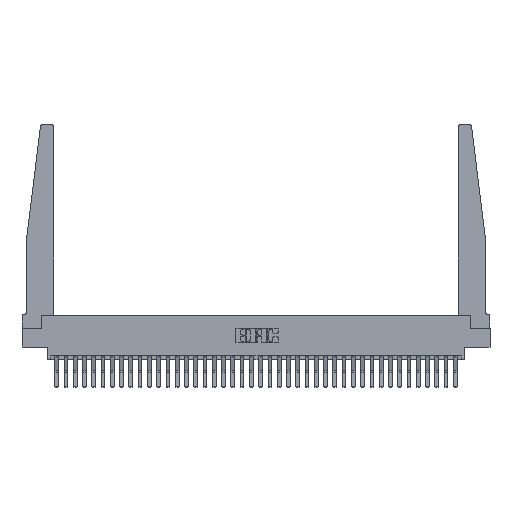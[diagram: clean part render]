
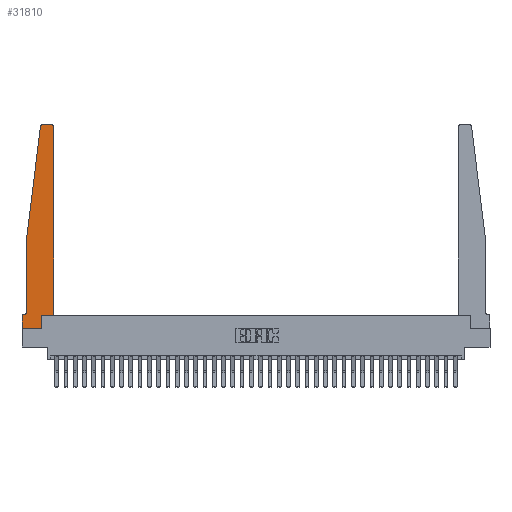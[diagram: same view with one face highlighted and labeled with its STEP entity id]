
A CAD part, top view. The second image highlights one B-rep face of the part: STEP entity #31810.
In plain terms, the highlighted planar face has unit normal (0, 0, 1).
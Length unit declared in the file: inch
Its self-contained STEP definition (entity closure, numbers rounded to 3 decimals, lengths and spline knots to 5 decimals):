
#384 = CARTESIAN_POINT ( 'NONE',  ( 0.2605, 0.18, 0.37 ) ) ;
#473 = DIRECTION ( 'NONE',  ( 1., 0., 0. ) ) ;
#571 = DIRECTION ( 'NONE',  ( 0., 0., -1. ) ) ;
#691 = AXIS2_PLACEMENT_3D ( 'NONE', #31772, #22110, #6333 ) ;
#906 = EDGE_CURVE ( 'NONE', #6547, #15479, #16368, .T. ) ;
#1162 = VERTEX_POINT ( 'NONE', #28659 ) ;
#2489 = LINE ( 'NONE', #23412, #5762 ) ;
#2725 = CARTESIAN_POINT ( 'NONE',  ( 0.27653, 2.75, 0.37 ) ) ;
#2829 = CARTESIAN_POINT ( 'NONE',  ( 0., 0., 0.37 ) ) ;
#3118 = EDGE_CURVE ( 'NONE', #28521, #12456, #17120, .T. ) ;
#3386 = VERTEX_POINT ( 'NONE', #4749 ) ;
#3524 = DIRECTION ( 'NONE',  ( 0., -1., 0. ) ) ;
#3864 = LINE ( 'NONE', #14000, #23705 ) ;
#3936 = EDGE_CURVE ( 'NONE', #12456, #9022, #10073, .T. ) ;
#4135 = VERTEX_POINT ( 'NONE', #10928 ) ;
#4567 = EDGE_CURVE ( 'NONE', #3386, #16780, #18551, .T. ) ;
#4601 = AXIS2_PLACEMENT_3D ( 'NONE', #26708, #16242, #473 ) ;
#4749 = CARTESIAN_POINT ( 'NONE',  ( 0.2605, 0., 0.37 ) ) ;
#4810 = EDGE_CURVE ( 'NONE', #9022, #14319, #25326, .T. ) ;
#5030 = ORIENTED_EDGE ( 'NONE', *, *, #12730, .T. ) ;
#5472 = EDGE_CURVE ( 'NONE', #22526, #6547, #3864, .T. ) ;
#5762 = VECTOR ( 'NONE', #27783, 39.37008 ) ;
#6156 = DIRECTION ( 'NONE',  ( -0.122, -0.992, 0. ) ) ;
#6333 = DIRECTION ( 'NONE',  ( 1., 0., 0. ) ) ;
#6546 = CARTESIAN_POINT ( 'NONE',  ( 0., 0.1875, 0.37 ) ) ;
#6547 = VERTEX_POINT ( 'NONE', #14654 ) ;
#6686 = AXIS2_PLACEMENT_3D ( 'NONE', #25741, #12544, #27960 ) ;
#6971 = VERTEX_POINT ( 'NONE', #6546 ) ;
#7208 = VECTOR ( 'NONE', #28725, 39.37008 ) ;
#7412 = CARTESIAN_POINT ( 'NONE',  ( 0., 0., 0.37 ) ) ;
#7685 = ORIENTED_EDGE ( 'NONE', *, *, #906, .T. ) ;
#8098 = DIRECTION ( 'NONE',  ( 1., 0., 0. ) ) ;
#8275 = ORIENTED_EDGE ( 'NONE', *, *, #3936, .T. ) ;
#8624 = CARTESIAN_POINT ( 'NONE',  ( 0.065, 1.25, 0.37 ) ) ;
#9022 = VERTEX_POINT ( 'NONE', #2725 ) ;
#9044 = ORIENTED_EDGE ( 'NONE', *, *, #3118, .T. ) ;
#9555 = ORIENTED_EDGE ( 'NONE', *, *, #17742, .T. ) ;
#10073 = LINE ( 'NONE', #28209, #7208 ) ;
#10223 = EDGE_CURVE ( 'NONE', #15479, #6971, #2489, .T. ) ;
#10928 = CARTESIAN_POINT ( 'NONE',  ( 0.425, 0.18, 0.37 ) ) ;
#11623 = CARTESIAN_POINT ( 'NONE',  ( 0.425, 2.72, 0.37 ) ) ;
#12456 = VERTEX_POINT ( 'NONE', #32374 ) ;
#12544 = DIRECTION ( 'NONE',  ( 0., 0., 1. ) ) ;
#12730 = EDGE_CURVE ( 'NONE', #6971, #1162, #20842, .T. ) ;
#13282 = EDGE_LOOP ( 'NONE', ( #8275, #27753, #20862, #17628, #7685, #32842, #5030, #33153, #15817, #9555, #27633, #9044 ) ) ;
#13893 = VECTOR ( 'NONE', #8098, 39.37008 ) ;
#13940 = CARTESIAN_POINT ( 'NONE',  ( 0.24675, 2.72367, 0.37 ) ) ;
#14000 = CARTESIAN_POINT ( 'NONE',  ( 0.065, 1.25, 0.37 ) ) ;
#14319 = VERTEX_POINT ( 'NONE', #13940 ) ;
#14654 = CARTESIAN_POINT ( 'NONE',  ( 0.065, 0.2375, 0.37 ) ) ;
#15479 = VERTEX_POINT ( 'NONE', #21376 ) ;
#15817 = ORIENTED_EDGE ( 'NONE', *, *, #4567, .T. ) ;
#16242 = DIRECTION ( 'NONE',  ( 0., 0., 1. ) ) ;
#16353 = DIRECTION ( 'NONE',  ( -1., 0., 0. ) ) ;
#16368 = CIRCLE ( 'NONE', #20175, 0.05 ) ;
#16486 = LINE ( 'NONE', #26950, #13893 ) ;
#16780 = VERTEX_POINT ( 'NONE', #33778 ) ;
#17120 = CIRCLE ( 'NONE', #691, 0.03 ) ;
#17628 = ORIENTED_EDGE ( 'NONE', *, *, #5472, .T. ) ;
#17742 = EDGE_CURVE ( 'NONE', #16780, #4135, #16486, .T. ) ;
#17862 = LINE ( 'NONE', #28661, #27159 ) ;
#17865 = DIRECTION ( 'NONE',  ( 1., 0., 0. ) ) ;
#18204 = VECTOR ( 'NONE', #6156, 39.37008 ) ;
#18551 = LINE ( 'NONE', #384, #26435 ) ;
#18797 = FACE_OUTER_BOUND ( 'NONE', #13282, .T. ) ;
#19353 = LINE ( 'NONE', #26912, #18204 ) ;
#20175 = AXIS2_PLACEMENT_3D ( 'NONE', #21840, #571, #16353 ) ;
#20842 = LINE ( 'NONE', #2829, #31060 ) ;
#20862 = ORIENTED_EDGE ( 'NONE', *, *, #30984, .T. ) ;
#21084 = EDGE_CURVE ( 'NONE', #4135, #28521, #17862, .T. ) ;
#21376 = CARTESIAN_POINT ( 'NONE',  ( 0.015, 0.1875, 0.37 ) ) ;
#21840 = CARTESIAN_POINT ( 'NONE',  ( 0.015, 0.2375, 0.37 ) ) ;
#22110 = DIRECTION ( 'NONE',  ( 0., 0., 1. ) ) ;
#22397 = EDGE_CURVE ( 'NONE', #1162, #3386, #25592, .T. ) ;
#22526 = VERTEX_POINT ( 'NONE', #8624 ) ;
#23412 = CARTESIAN_POINT ( 'NONE',  ( 0.065, 0.1875, 0.37 ) ) ;
#23705 = VECTOR ( 'NONE', #3524, 39.37008 ) ;
#25326 = CIRCLE ( 'NONE', #6686, 0.03 ) ;
#25560 = VECTOR ( 'NONE', #17865, 39.37008 ) ;
#25592 = LINE ( 'NONE', #7412, #25560 ) ;
#25741 = CARTESIAN_POINT ( 'NONE',  ( 0.27653, 2.72, 0.37 ) ) ;
#25926 = DIRECTION ( 'NONE',  ( 0., 1., 0. ) ) ;
#26435 = VECTOR ( 'NONE', #26623, 39.37008 ) ;
#26623 = DIRECTION ( 'NONE',  ( 0., 1., 0. ) ) ;
#26708 = CARTESIAN_POINT ( 'NONE',  ( 0., 0.1875, 0.37 ) ) ;
#26912 = CARTESIAN_POINT ( 'NONE',  ( 0.065, 1.25, 0.37 ) ) ;
#26950 = CARTESIAN_POINT ( 'NONE',  ( 0.425, 0.18, 0.37 ) ) ;
#27159 = VECTOR ( 'NONE', #25926, 39.37008 ) ;
#27633 = ORIENTED_EDGE ( 'NONE', *, *, #21084, .T. ) ;
#27753 = ORIENTED_EDGE ( 'NONE', *, *, #4810, .T. ) ;
#27783 = DIRECTION ( 'NONE',  ( -1., 0., 0. ) ) ;
#27960 = DIRECTION ( 'NONE',  ( 1., 0., 0. ) ) ;
#28209 = CARTESIAN_POINT ( 'NONE',  ( 0.25, 2.75, 0.37 ) ) ;
#28521 = VERTEX_POINT ( 'NONE', #11623 ) ;
#28659 = CARTESIAN_POINT ( 'NONE',  ( 0., 0., 0.37 ) ) ;
#28661 = CARTESIAN_POINT ( 'NONE',  ( 0.425, 0.18, 0.37 ) ) ;
#28725 = DIRECTION ( 'NONE',  ( -1., 0., 0. ) ) ;
#30984 = EDGE_CURVE ( 'NONE', #14319, #22526, #19353, .T. ) ;
#31060 = VECTOR ( 'NONE', #31297, 39.37008 ) ;
#31297 = DIRECTION ( 'NONE',  ( 0., -1., 0. ) ) ;
#31513 = PLANE ( 'NONE',  #4601 ) ;
#31772 = CARTESIAN_POINT ( 'NONE',  ( 0.395, 2.72, 0.37 ) ) ;
#31810 = ADVANCED_FACE ( 'NONE', ( #18797 ), #31513, .T. ) ;
#32374 = CARTESIAN_POINT ( 'NONE',  ( 0.395, 2.75, 0.37 ) ) ;
#32842 = ORIENTED_EDGE ( 'NONE', *, *, #10223, .T. ) ;
#33153 = ORIENTED_EDGE ( 'NONE', *, *, #22397, .T. ) ;
#33778 = CARTESIAN_POINT ( 'NONE',  ( 0.2605, 0.18, 0.37 ) ) ;
